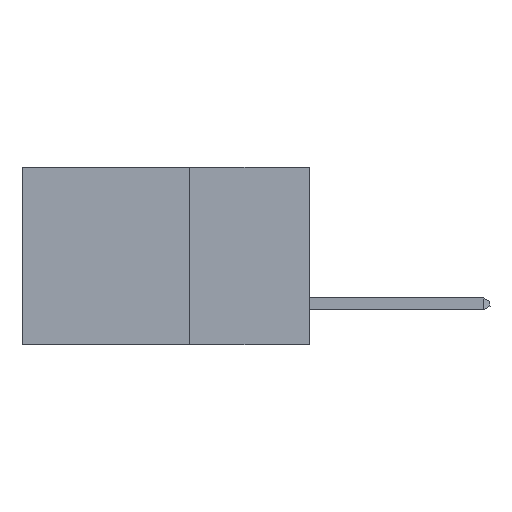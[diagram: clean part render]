
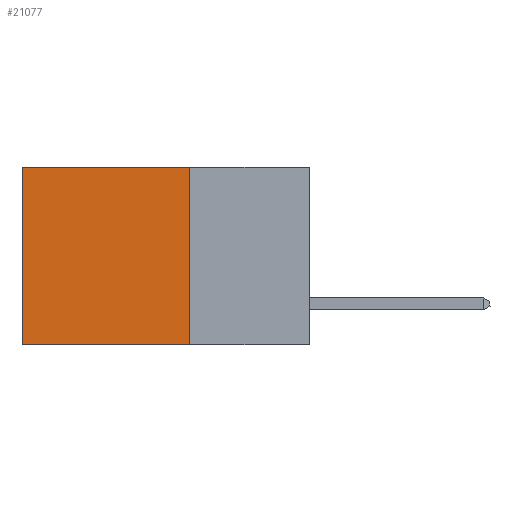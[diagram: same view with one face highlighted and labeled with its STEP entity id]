
A CAD part, left-side view. The second image highlights one B-rep face of the part: STEP entity #21077.
In plain terms, the highlighted planar face has unit normal (-1, 0, 0).
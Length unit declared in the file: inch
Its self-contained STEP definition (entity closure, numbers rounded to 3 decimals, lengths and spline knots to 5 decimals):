
#183 = CARTESIAN_POINT ( 'NONE',  ( 0.2875, 0.25, 0. ) ) ;
#419 = LINE ( 'NONE', #15861, #22262 ) ;
#602 = VECTOR ( 'NONE', #14568, 39.37008 ) ;
#642 = ORIENTED_EDGE ( 'NONE', *, *, #17111, .T. ) ;
#773 = VERTEX_POINT ( 'NONE', #7665 ) ;
#1947 = CARTESIAN_POINT ( 'NONE',  ( 0.2875, 0.25, 0. ) ) ;
#2846 = VECTOR ( 'NONE', #20600, 39.37008 ) ;
#2895 = LINE ( 'NONE', #183, #11668 ) ;
#6704 = AXIS2_PLACEMENT_3D ( 'NONE', #15675, #20701, #10662 ) ;
#6724 = EDGE_CURVE ( 'NONE', #18846, #15100, #2895, .T. ) ;
#7424 = ORIENTED_EDGE ( 'NONE', *, *, #12762, .F. ) ;
#7665 = CARTESIAN_POINT ( 'NONE',  ( 0.2875, 0.6, 0. ) ) ;
#7803 = EDGE_LOOP ( 'NONE', ( #8497, #7424, #10423, #642 ) ) ;
#8497 = ORIENTED_EDGE ( 'NONE', *, *, #15552, .T. ) ;
#8521 = FACE_OUTER_BOUND ( 'NONE', #7803, .T. ) ;
#8987 = PLANE ( 'NONE',  #6704 ) ;
#10113 = LINE ( 'NONE', #12844, #602 ) ;
#10423 = ORIENTED_EDGE ( 'NONE', *, *, #6724, .F. ) ;
#10662 = DIRECTION ( 'NONE',  ( 0., 0., -1. ) ) ;
#10849 = DIRECTION ( 'NONE',  ( 0., 1., 0. ) ) ;
#11625 = LINE ( 'NONE', #18936, #2846 ) ;
#11668 = VECTOR ( 'NONE', #12586, 39.37008 ) ;
#12586 = DIRECTION ( 'NONE',  ( 0., 0., -1. ) ) ;
#12762 = EDGE_CURVE ( 'NONE', #15100, #20506, #419, .T. ) ;
#12844 = CARTESIAN_POINT ( 'NONE',  ( 0.2875, 0.6, 0. ) ) ;
#13624 = CARTESIAN_POINT ( 'NONE',  ( 0.2875, 0.6, -0.37 ) ) ;
#14568 = DIRECTION ( 'NONE',  ( 0., 0., -1. ) ) ;
#15100 = VERTEX_POINT ( 'NONE', #16599 ) ;
#15552 = EDGE_CURVE ( 'NONE', #773, #20506, #10113, .T. ) ;
#15675 = CARTESIAN_POINT ( 'NONE',  ( 0.2875, 0.25, 0. ) ) ;
#15861 = CARTESIAN_POINT ( 'NONE',  ( 0.2875, 0.25, -0.37 ) ) ;
#16599 = CARTESIAN_POINT ( 'NONE',  ( 0.2875, 0.25, -0.37 ) ) ;
#17111 = EDGE_CURVE ( 'NONE', #18846, #773, #11625, .T. ) ;
#18846 = VERTEX_POINT ( 'NONE', #1947 ) ;
#18936 = CARTESIAN_POINT ( 'NONE',  ( 0.2875, 0.25, 0. ) ) ;
#20506 = VERTEX_POINT ( 'NONE', #13624 ) ;
#20600 = DIRECTION ( 'NONE',  ( 0., 1., 0. ) ) ;
#20701 = DIRECTION ( 'NONE',  ( 1., 0., 0. ) ) ;
#21077 = ADVANCED_FACE ( 'NONE', ( #8521 ), #8987, .F. ) ;
#22262 = VECTOR ( 'NONE', #10849, 39.37008 ) ;
